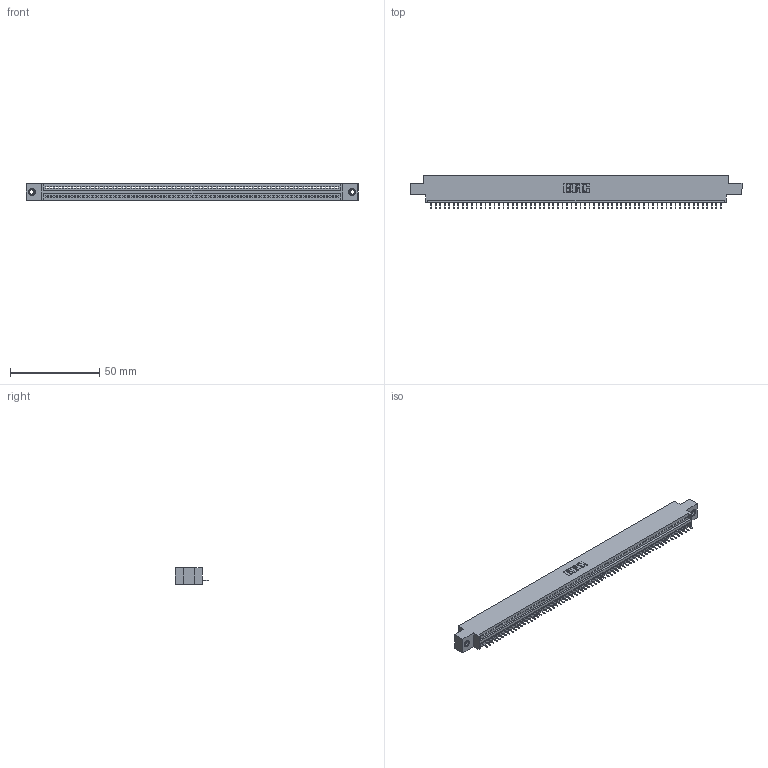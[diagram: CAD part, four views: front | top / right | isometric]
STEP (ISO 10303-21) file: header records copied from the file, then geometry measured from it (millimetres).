
FILE_DESCRIPTION (( 'STEP AP203' ), '1' );
FILE_NAME ('845-065-525-607.STEP', '2020-09-23T18:42:09', ( '' ), ( '' ), 'SwSTEP 2.0', 'SolidWorks 2020', '' );
FILE_SCHEMA (( 'CONFIG_CONTROL_DESIGN' ));
Length unit declared in the file: inch
Products named in the file (4): 345-250-001_345-250-005-103; 845-065-525-607; 845 Part_0.170 Offset - 0.156 Dia-TI; 345-292-001_345-293-125
Assembly tree (68 placements, depth 2):
  845-065-525-607
    845 Part_0.170 Offset - 0.156 Dia-TI
    345-292-001_345-293-125  x65
    345-250-001_345-250-005-103  x2
Bounding box: 186.31 x 18.72 x 9.4 mm (x, y, z)
Volume: 17491.9 mm3; surface area: 22831.9 mm2
Topology: 68 solids, 68 shells, 4220 faces, 12189 edges, 7858 vertices
Faces by surface type: plane 3106, cylinder 1098, cone 12, torus 4
Entity records: 47216 total; most frequent: CARTESIAN_POINT 8158, ORIENTED_EDGE 8150, DIRECTION 7119, EDGE_CURVE 4075, LINE 3667, VECTOR 3667, VERTEX_POINT 2708, AXIS2_PLACEMENT_3D 1726
